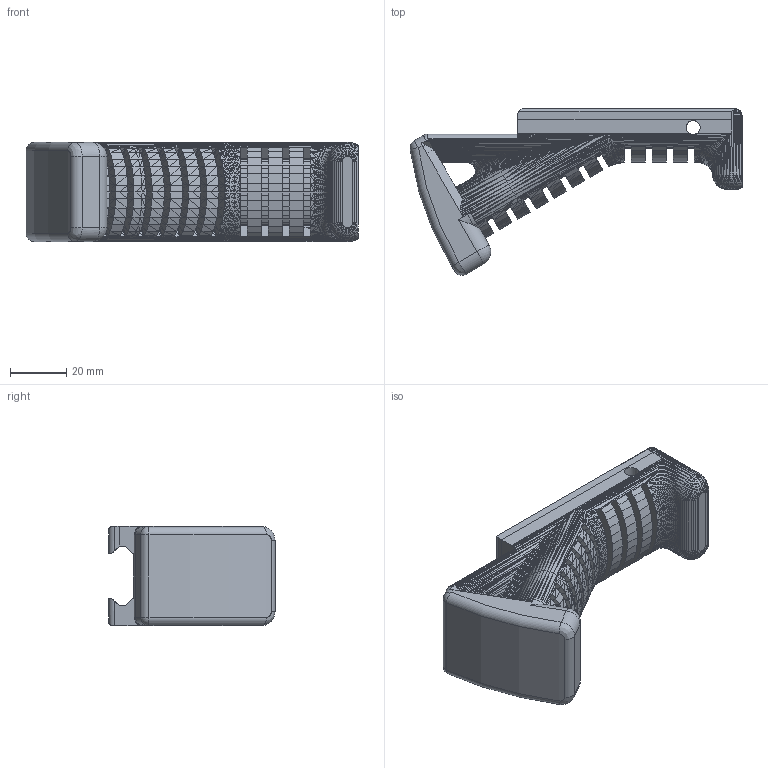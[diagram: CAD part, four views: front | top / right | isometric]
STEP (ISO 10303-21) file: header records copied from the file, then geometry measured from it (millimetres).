
FILE_DESCRIPTION(/* description */ (''),/* implementation_level */ '2;1');
FILE_NAME(/* name */ 'vz61 AFG.step',/* time_stamp */ '2021-02-09T08:47:09-07:00',/* author */ (''),/* organization */ (''),/* preprocessor_version */ 'ST-DEVELOPER v18.1',/* originating_system */ 'Autodesk Translation Framework v9.7.1.1290',/* authorisation */ '');
FILE_SCHEMA (('AUTOMOTIVE_DESIGN { 1 0 10303 214 3 1 1 }'));
Length unit declared in the file: millimetre
Products named in the file (1): vz61 Handguard
Bounding box: 118.52 x 59.43 x 35.41 mm (x, y, z)
Volume: 87707.5 mm3; surface area: 24412.5 mm2
Topology: 2 solids, 2 shells, 5677 faces, 9272 edges, 3592 vertices
Faces by surface type: plane 5639, cylinder 22, bspline 8, sphere 6, torus 2
Full cylindrical faces by diameter (mm): 5 x1
Entity records: 117874 total; most frequent: DIRECTION 20722, CARTESIAN_POINT 18798, ORIENTED_EDGE 18544, EDGE_CURVE 9272, LINE 9106, VECTOR 9106, AXIS2_PLACEMENT_3D 5808, EDGE_LOOP 5678
